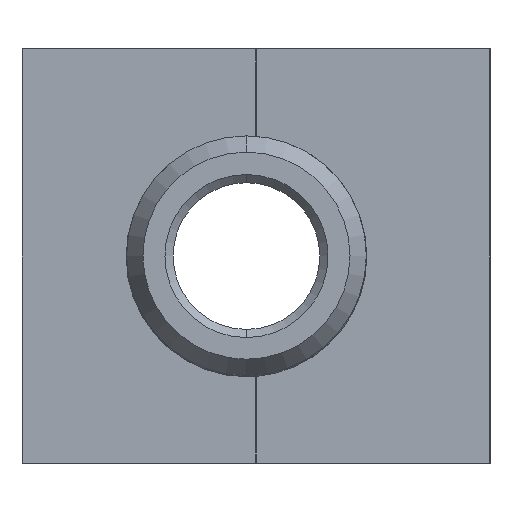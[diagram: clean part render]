
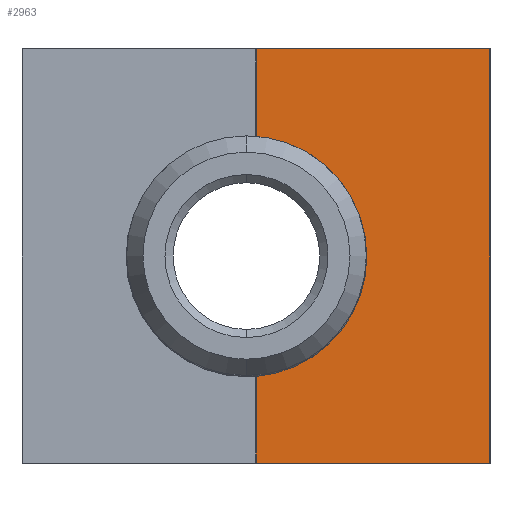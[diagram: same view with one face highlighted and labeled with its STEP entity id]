
A CAD part, left-side view. The second image highlights one B-rep face of the part: STEP entity #2963.
In plain terms, the highlighted face is planar.
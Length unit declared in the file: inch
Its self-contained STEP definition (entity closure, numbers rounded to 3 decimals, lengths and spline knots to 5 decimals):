
#262 = LINE ( 'NONE', #16914, #11696 ) ;
#1439 = LINE ( 'NONE', #7122, #18255 ) ;
#1940 = AXIS2_PLACEMENT_3D ( 'NONE', #14285, #11528, #14573 ) ;
#2752 = PLANE ( 'NONE',  #2859 ) ;
#2859 = AXIS2_PLACEMENT_3D ( 'NONE', #16002, #8445, #14713 ) ;
#2963 = ADVANCED_FACE ( 'NONE', ( #11579 ), #2752, .F. ) ;
#3187 = ORIENTED_EDGE ( 'NONE', *, *, #16133, .F. ) ;
#3368 = CARTESIAN_POINT ( 'NONE',  ( 0., -1.13, 0. ) ) ;
#3624 = CARTESIAN_POINT ( 'NONE',  ( 0., -1.13, 0. ) ) ;
#3918 = EDGE_CURVE ( 'NONE', #4355, #7980, #10705, .T. ) ;
#4355 = VERTEX_POINT ( 'NONE', #13166 ) ;
#4552 = CARTESIAN_POINT ( 'NONE',  ( 0., 0., 0. ) ) ;
#4835 = CARTESIAN_POINT ( 'NONE',  ( 0.79065, -0.565, 0. ) ) ;
#4901 = EDGE_CURVE ( 'NONE', #18927, #5092, #1439, .T. ) ;
#5092 = VERTEX_POINT ( 'NONE', #6438 ) ;
#5240 = ORIENTED_EDGE ( 'NONE', *, *, #5836, .T. ) ;
#5836 = EDGE_CURVE ( 'NONE', #14724, #4355, #10701, .T. ) ;
#6137 = LINE ( 'NONE', #4552, #8470 ) ;
#6195 = CARTESIAN_POINT ( 'NONE',  ( 0., -0.565, 0. ) ) ;
#6438 = CARTESIAN_POINT ( 'NONE',  ( 1., -0.565, 0. ) ) ;
#6861 = EDGE_CURVE ( 'NONE', #14724, #12848, #6137, .T. ) ;
#7122 = CARTESIAN_POINT ( 'NONE',  ( 1., 0., 0. ) ) ;
#7320 = DIRECTION ( 'NONE',  ( 0., 1., 0. ) ) ;
#7631 = VECTOR ( 'NONE', #17855, 39.37008 ) ;
#7980 = VERTEX_POINT ( 'NONE', #4835 ) ;
#8445 = DIRECTION ( 'NONE',  ( 0., 0., 1. ) ) ;
#8470 = VECTOR ( 'NONE', #15160, 39.37008 ) ;
#9351 = DIRECTION ( 'NONE',  ( 1., 0., 0. ) ) ;
#10567 = CARTESIAN_POINT ( 'NONE',  ( 1., -1.13, 0. ) ) ;
#10701 = LINE ( 'NONE', #6195, #7631 ) ;
#10705 = CIRCLE ( 'NONE', #1940, 0.29055 ) ;
#10842 = DIRECTION ( 'NONE',  ( 1., 0., 0. ) ) ;
#11019 = EDGE_CURVE ( 'NONE', #7980, #5092, #262, .T. ) ;
#11528 = DIRECTION ( 'NONE',  ( 0., 0., 1. ) ) ;
#11579 = FACE_OUTER_BOUND ( 'NONE', #15282, .T. ) ;
#11696 = VECTOR ( 'NONE', #10842, 39.37008 ) ;
#12293 = LINE ( 'NONE', #3368, #17757 ) ;
#12848 = VERTEX_POINT ( 'NONE', #3624 ) ;
#13166 = CARTESIAN_POINT ( 'NONE',  ( 0.21138, -0.565, 0. ) ) ;
#13422 = ORIENTED_EDGE ( 'NONE', *, *, #4901, .F. ) ;
#13953 = CARTESIAN_POINT ( 'NONE',  ( 0., -0.565, 0. ) ) ;
#14079 = ORIENTED_EDGE ( 'NONE', *, *, #6861, .F. ) ;
#14143 = ORIENTED_EDGE ( 'NONE', *, *, #3918, .T. ) ;
#14285 = CARTESIAN_POINT ( 'NONE',  ( 0.50101, -0.54197, 0. ) ) ;
#14573 = DIRECTION ( 'NONE',  ( 1., 0., 0. ) ) ;
#14713 = DIRECTION ( 'NONE',  ( 1., 0., 0. ) ) ;
#14724 = VERTEX_POINT ( 'NONE', #13953 ) ;
#14835 = ORIENTED_EDGE ( 'NONE', *, *, #11019, .T. ) ;
#15160 = DIRECTION ( 'NONE',  ( 0., -1., 0. ) ) ;
#15282 = EDGE_LOOP ( 'NONE', ( #14079, #5240, #14143, #14835, #13422, #3187 ) ) ;
#16002 = CARTESIAN_POINT ( 'NONE',  ( 0., 0., 0. ) ) ;
#16133 = EDGE_CURVE ( 'NONE', #12848, #18927, #12293, .T. ) ;
#16914 = CARTESIAN_POINT ( 'NONE',  ( 0., -0.565, 0. ) ) ;
#17757 = VECTOR ( 'NONE', #9351, 39.37008 ) ;
#17855 = DIRECTION ( 'NONE',  ( 1., 0., 0. ) ) ;
#18255 = VECTOR ( 'NONE', #7320, 39.37008 ) ;
#18927 = VERTEX_POINT ( 'NONE', #10567 ) ;
